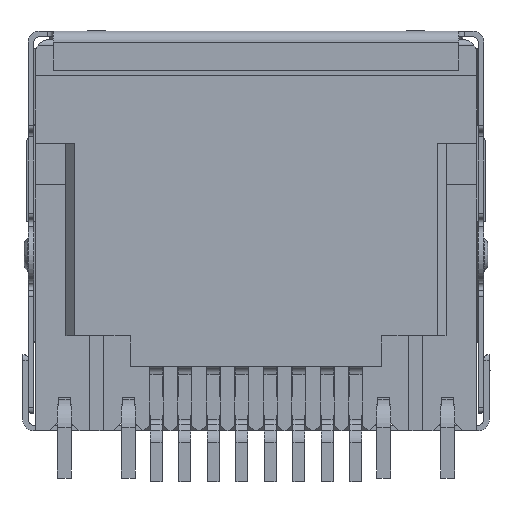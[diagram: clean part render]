
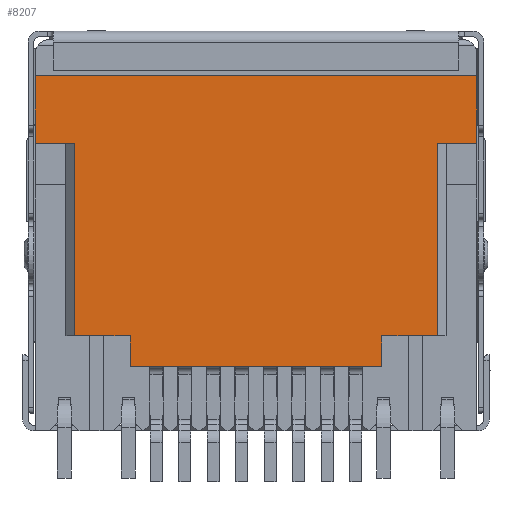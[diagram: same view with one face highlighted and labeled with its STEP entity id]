
A CAD part, front view. The second image highlights one B-rep face of the part: STEP entity #8207.
In plain terms, the highlighted planar face has unit normal (0, -1, 0).
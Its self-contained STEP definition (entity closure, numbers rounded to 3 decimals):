
#189 = CARTESIAN_POINT ( 'NONE',  ( -7.9, -5.525, -10.6 ) ) ;
#1812 = DIRECTION ( 'NONE',  ( 0., 0., -1. ) ) ;
#1837 = DIRECTION ( 'NONE',  ( -1., 0., 0. ) ) ;
#2159 = LINE ( 'NONE', #189, #8836 ) ;
#2536 = EDGE_CURVE ( 'NONE', #29905, #44009, #22425, .T. ) ;
#2810 = VERTEX_POINT ( 'NONE', #8791 ) ;
#2853 = ORIENTED_EDGE ( 'NONE', *, *, #9958, .F. ) ;
#3867 = VECTOR ( 'NONE', #33274, 1000. ) ;
#3872 = CARTESIAN_POINT ( 'NONE',  ( 6.5, -5.525, -3.7 ) ) ;
#3993 = CARTESIAN_POINT ( 'NONE',  ( -7.9, -5.525, -11.7 ) ) ;
#4935 = VERTEX_POINT ( 'NONE', #35304 ) ;
#5063 = CARTESIAN_POINT ( 'NONE',  ( 7.9, -5.525, -14. ) ) ;
#5079 = DIRECTION ( 'NONE',  ( 0., 0., 1. ) ) ;
#5086 = LINE ( 'NONE', #41029, #8076 ) ;
#5222 = ORIENTED_EDGE ( 'NONE', *, *, #45828, .T. ) ;
#5559 = EDGE_CURVE ( 'NONE', #35360, #4935, #40312, .T. ) ;
#5808 = CARTESIAN_POINT ( 'NONE',  ( 4.5, -5.525, -10.6 ) ) ;
#6055 = CARTESIAN_POINT ( 'NONE',  ( 4.5, -5.525, -10.6 ) ) ;
#6093 = LINE ( 'NONE', #7876, #10312 ) ;
#7876 = CARTESIAN_POINT ( 'NONE',  ( -7.9, -5.525, -14. ) ) ;
#8076 = VECTOR ( 'NONE', #1837, 1000. ) ;
#8207 = ADVANCED_FACE ( 'NONE', ( #19420 ), #35480, .T. ) ;
#8791 = CARTESIAN_POINT ( 'NONE',  ( -7.9, -5.525, -3.7 ) ) ;
#8836 = VECTOR ( 'NONE', #20399, 1000. ) ;
#9466 = CARTESIAN_POINT ( 'NONE',  ( 6.5, -5.525, -14. ) ) ;
#9497 = DIRECTION ( 'NONE',  ( 0., 0., -1. ) ) ;
#9958 = EDGE_CURVE ( 'NONE', #2810, #47387, #6093, .T. ) ;
#10312 = VECTOR ( 'NONE', #11965, 1000. ) ;
#10556 = LINE ( 'NONE', #25946, #45199 ) ;
#10682 = VERTEX_POINT ( 'NONE', #23442 ) ;
#10968 = ORIENTED_EDGE ( 'NONE', *, *, #31599, .T. ) ;
#11965 = DIRECTION ( 'NONE',  ( 0., 0., 1. ) ) ;
#12058 = ORIENTED_EDGE ( 'NONE', *, *, #33279, .T. ) ;
#12148 = ORIENTED_EDGE ( 'NONE', *, *, #42635, .T. ) ;
#13117 = CARTESIAN_POINT ( 'NONE',  ( -4.5, -5.525, -10.6 ) ) ;
#14747 = LINE ( 'NONE', #5063, #30454 ) ;
#14788 = VECTOR ( 'NONE', #34710, 1000. ) ;
#15084 = EDGE_CURVE ( 'NONE', #10682, #4935, #14747, .T. ) ;
#16785 = CARTESIAN_POINT ( 'NONE',  ( 6.5, -5.525, -10.6 ) ) ;
#17272 = LINE ( 'NONE', #13117, #36107 ) ;
#18136 = DIRECTION ( 'NONE',  ( 1., 0., 0. ) ) ;
#18784 = ORIENTED_EDGE ( 'NONE', *, *, #24981, .T. ) ;
#19420 = FACE_OUTER_BOUND ( 'NONE', #47071, .T. ) ;
#19752 = ORIENTED_EDGE ( 'NONE', *, *, #46149, .T. ) ;
#20399 = DIRECTION ( 'NONE',  ( 1., 0., 0. ) ) ;
#20901 = DIRECTION ( 'NONE',  ( 0., -1., 0. ) ) ;
#21513 = LINE ( 'NONE', #5808, #3867 ) ;
#22425 = LINE ( 'NONE', #49935, #27850 ) ;
#23201 = CARTESIAN_POINT ( 'NONE',  ( -4.5, -5.525, -10.6 ) ) ;
#23442 = CARTESIAN_POINT ( 'NONE',  ( 7.9, -5.525, -1.3 ) ) ;
#24466 = ORIENTED_EDGE ( 'NONE', *, *, #38568, .T. ) ;
#24981 = EDGE_CURVE ( 'NONE', #10682, #47387, #5086, .T. ) ;
#25783 = DIRECTION ( 'NONE',  ( 1., 0., 0. ) ) ;
#25946 = CARTESIAN_POINT ( 'NONE',  ( -7.9, -5.525, -10.6 ) ) ;
#26589 = DIRECTION ( 'NONE',  ( 0., 0., -1. ) ) ;
#26902 = CARTESIAN_POINT ( 'NONE',  ( -7.9, -5.525, -3.7 ) ) ;
#27536 = VERTEX_POINT ( 'NONE', #6055 ) ;
#27850 = VECTOR ( 'NONE', #26589, 1000. ) ;
#28457 = CARTESIAN_POINT ( 'NONE',  ( -6.5, -5.525, -10.6 ) ) ;
#28929 = VERTEX_POINT ( 'NONE', #35142 ) ;
#29065 = CARTESIAN_POINT ( 'NONE',  ( -6.5, -5.525, -3.7 ) ) ;
#29905 = VERTEX_POINT ( 'NONE', #29065 ) ;
#30454 = VECTOR ( 'NONE', #1812, 1000. ) ;
#30804 = DIRECTION ( 'NONE',  ( 1., 0., 0. ) ) ;
#31599 = EDGE_CURVE ( 'NONE', #44009, #37758, #2159, .T. ) ;
#33248 = ORIENTED_EDGE ( 'NONE', *, *, #5559, .T. ) ;
#33274 = DIRECTION ( 'NONE',  ( 0., 0., 1. ) ) ;
#33279 = EDGE_CURVE ( 'NONE', #27536, #45812, #10556, .T. ) ;
#34710 = DIRECTION ( 'NONE',  ( 1., 0., 0. ) ) ;
#35142 = CARTESIAN_POINT ( 'NONE',  ( -4.5, -5.525, -11.7 ) ) ;
#35304 = CARTESIAN_POINT ( 'NONE',  ( 7.9, -5.525, -3.7 ) ) ;
#35360 = VERTEX_POINT ( 'NONE', #3872 ) ;
#35480 = PLANE ( 'NONE',  #37446 ) ;
#36107 = VECTOR ( 'NONE', #48106, 1000. ) ;
#36518 = CARTESIAN_POINT ( 'NONE',  ( 4.5, -5.525, -11.7 ) ) ;
#36884 = ORIENTED_EDGE ( 'NONE', *, *, #41277, .T. ) ;
#37446 = AXIS2_PLACEMENT_3D ( 'NONE', #46884, #20901, #9497 ) ;
#37727 = VECTOR ( 'NONE', #30804, 1000. ) ;
#37758 = VERTEX_POINT ( 'NONE', #23201 ) ;
#38203 = ORIENTED_EDGE ( 'NONE', *, *, #15084, .F. ) ;
#38568 = EDGE_CURVE ( 'NONE', #43618, #27536, #21513, .T. ) ;
#40312 = LINE ( 'NONE', #26902, #14788 ) ;
#40630 = VECTOR ( 'NONE', #18136, 1000. ) ;
#41029 = CARTESIAN_POINT ( 'NONE',  ( -7.9, -5.525, -1.3 ) ) ;
#41277 = EDGE_CURVE ( 'NONE', #37758, #28929, #17272, .T. ) ;
#41368 = CARTESIAN_POINT ( 'NONE',  ( -7.9, -5.525, -3.7 ) ) ;
#41413 = VECTOR ( 'NONE', #5079, 1000. ) ;
#42635 = EDGE_CURVE ( 'NONE', #2810, #29905, #46104, .T. ) ;
#43618 = VERTEX_POINT ( 'NONE', #36518 ) ;
#44009 = VERTEX_POINT ( 'NONE', #28457 ) ;
#45199 = VECTOR ( 'NONE', #25783, 1000. ) ;
#45677 = LINE ( 'NONE', #9466, #41413 ) ;
#45812 = VERTEX_POINT ( 'NONE', #16785 ) ;
#45828 = EDGE_CURVE ( 'NONE', #45812, #35360, #45677, .T. ) ;
#46041 = CARTESIAN_POINT ( 'NONE',  ( -7.9, -5.525, -1.3 ) ) ;
#46104 = LINE ( 'NONE', #41368, #40630 ) ;
#46149 = EDGE_CURVE ( 'NONE', #28929, #43618, #49313, .T. ) ;
#46884 = CARTESIAN_POINT ( 'NONE',  ( -7.9, -5.525, -14. ) ) ;
#47071 = EDGE_LOOP ( 'NONE', ( #33248, #38203, #18784, #2853, #12148, #49612, #10968, #36884, #19752, #24466, #12058, #5222 ) ) ;
#47387 = VERTEX_POINT ( 'NONE', #46041 ) ;
#48106 = DIRECTION ( 'NONE',  ( 0., 0., -1. ) ) ;
#49313 = LINE ( 'NONE', #3993, #37727 ) ;
#49612 = ORIENTED_EDGE ( 'NONE', *, *, #2536, .T. ) ;
#49935 = CARTESIAN_POINT ( 'NONE',  ( -6.5, -5.525, -14. ) ) ;
